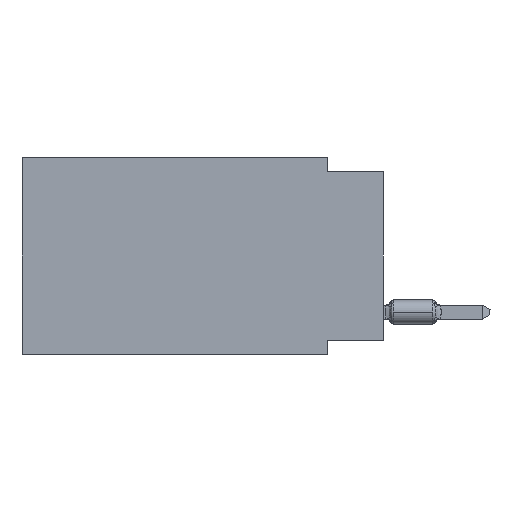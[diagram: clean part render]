
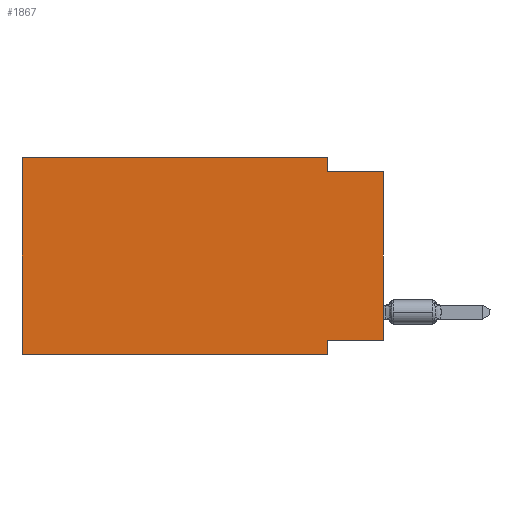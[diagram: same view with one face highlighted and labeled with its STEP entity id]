
A CAD part, left-side view. The second image highlights one B-rep face of the part: STEP entity #1867.
In plain terms, the highlighted planar face has unit normal (-1, 0, 0).
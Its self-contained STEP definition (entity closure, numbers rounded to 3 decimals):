
#154 = LINE ( 'NONE', #67499, #51391 ) ;
#655 = CARTESIAN_POINT ( 'NONE',  ( 0., 2.54, -0.635 ) ) ;
#1867 = ADVANCED_FACE ( 'NONE', ( #7643 ), #2832, .F. ) ;
#2832 = PLANE ( 'NONE',  #65739 ) ;
#3034 = EDGE_CURVE ( 'NONE', #3789, #51881, #59433, .T. ) ;
#3789 = VERTEX_POINT ( 'NONE', #67190 ) ;
#3911 = DIRECTION ( 'NONE',  ( 0., -1., 0. ) ) ;
#4207 = DIRECTION ( 'NONE',  ( 0., -1., 0. ) ) ;
#5122 = CARTESIAN_POINT ( 'NONE',  ( 0., 16.383, 0. ) ) ;
#7643 = FACE_OUTER_BOUND ( 'NONE', #57859, .T. ) ;
#7792 = EDGE_CURVE ( 'NONE', #61002, #53414, #52533, .T. ) ;
#8003 = EDGE_CURVE ( 'NONE', #22742, #40839, #56196, .T. ) ;
#10367 = VECTOR ( 'NONE', #4207, 1000. ) ;
#12188 = EDGE_CURVE ( 'NONE', #40839, #38805, #57077, .T. ) ;
#13279 = VECTOR ( 'NONE', #58087, 1000. ) ;
#13514 = CARTESIAN_POINT ( 'NONE',  ( 0., 16.383, 0. ) ) ;
#16881 = ORIENTED_EDGE ( 'NONE', *, *, #3034, .T. ) ;
#18961 = CARTESIAN_POINT ( 'NONE',  ( 0., 2.54, 0. ) ) ;
#22253 = DIRECTION ( 'NONE',  ( 0., 0., 1. ) ) ;
#22742 = VERTEX_POINT ( 'NONE', #44906 ) ;
#22993 = CARTESIAN_POINT ( 'NONE',  ( 0., 2.54, -8.89 ) ) ;
#23925 = CARTESIAN_POINT ( 'NONE',  ( 0., 0., -0.635 ) ) ;
#24015 = EDGE_CURVE ( 'NONE', #38805, #30561, #26499, .T. ) ;
#26151 = CARTESIAN_POINT ( 'NONE',  ( 0., 2.54, 0. ) ) ;
#26499 = LINE ( 'NONE', #26151, #55905 ) ;
#29197 = ORIENTED_EDGE ( 'NONE', *, *, #32915, .F. ) ;
#30561 = VERTEX_POINT ( 'NONE', #655 ) ;
#32915 = EDGE_CURVE ( 'NONE', #30561, #51881, #44941, .T. ) ;
#32962 = CARTESIAN_POINT ( 'NONE',  ( 0., 16.383, 0. ) ) ;
#33494 = CARTESIAN_POINT ( 'NONE',  ( 0., 0., 0. ) ) ;
#38802 = EDGE_CURVE ( 'NONE', #22742, #53414, #51077, .T. ) ;
#38805 = VERTEX_POINT ( 'NONE', #18961 ) ;
#40839 = VERTEX_POINT ( 'NONE', #63967 ) ;
#41235 = CARTESIAN_POINT ( 'NONE',  ( 0., 2.54, -8.89 ) ) ;
#41567 = CARTESIAN_POINT ( 'NONE',  ( 0., 2.54, -8.255 ) ) ;
#41884 = DIRECTION ( 'NONE',  ( 0., 1., 0. ) ) ;
#42263 = DIRECTION ( 'NONE',  ( 0., 0., -1. ) ) ;
#42413 = VECTOR ( 'NONE', #42263, 1000. ) ;
#43211 = DIRECTION ( 'NONE',  ( 1., 0., 0. ) ) ;
#44906 = CARTESIAN_POINT ( 'NONE',  ( 0., 16.383, -8.89 ) ) ;
#44941 = LINE ( 'NONE', #65782, #63286 ) ;
#46166 = ORIENTED_EDGE ( 'NONE', *, *, #8003, .F. ) ;
#46288 = DIRECTION ( 'NONE',  ( 0., 0., -1. ) ) ;
#51077 = LINE ( 'NONE', #60277, #10367 ) ;
#51214 = VECTOR ( 'NONE', #56529, 1000. ) ;
#51391 = VECTOR ( 'NONE', #41884, 1000. ) ;
#51881 = VERTEX_POINT ( 'NONE', #23925 ) ;
#52533 = LINE ( 'NONE', #41235, #42413 ) ;
#53342 = ORIENTED_EDGE ( 'NONE', *, *, #7792, .F. ) ;
#53414 = VERTEX_POINT ( 'NONE', #22993 ) ;
#53476 = ORIENTED_EDGE ( 'NONE', *, *, #12188, .F. ) ;
#55905 = VECTOR ( 'NONE', #46288, 1000. ) ;
#56196 = LINE ( 'NONE', #13514, #51214 ) ;
#56529 = DIRECTION ( 'NONE',  ( 0., 0., 1. ) ) ;
#57077 = LINE ( 'NONE', #5122, #13279 ) ;
#57480 = EDGE_CURVE ( 'NONE', #3789, #61002, #154, .T. ) ;
#57859 = EDGE_LOOP ( 'NONE', ( #16881, #29197, #62377, #53476, #46166, #60210, #53342, #62595 ) ) ;
#58087 = DIRECTION ( 'NONE',  ( 0., -1., 0. ) ) ;
#59433 = LINE ( 'NONE', #33494, #61640 ) ;
#60210 = ORIENTED_EDGE ( 'NONE', *, *, #38802, .T. ) ;
#60277 = CARTESIAN_POINT ( 'NONE',  ( 0., 16.383, -8.89 ) ) ;
#61002 = VERTEX_POINT ( 'NONE', #41567 ) ;
#61640 = VECTOR ( 'NONE', #22253, 1000. ) ;
#62377 = ORIENTED_EDGE ( 'NONE', *, *, #24015, .F. ) ;
#62595 = ORIENTED_EDGE ( 'NONE', *, *, #57480, .F. ) ;
#63286 = VECTOR ( 'NONE', #3911, 1000. ) ;
#63967 = CARTESIAN_POINT ( 'NONE',  ( 0., 16.383, 0. ) ) ;
#64382 = DIRECTION ( 'NONE',  ( 0., 0., -1. ) ) ;
#65739 = AXIS2_PLACEMENT_3D ( 'NONE', #32962, #43211, #64382 ) ;
#65782 = CARTESIAN_POINT ( 'NONE',  ( 0., 0., -0.635 ) ) ;
#67190 = CARTESIAN_POINT ( 'NONE',  ( 0., 0., -8.255 ) ) ;
#67499 = CARTESIAN_POINT ( 'NONE',  ( 0., 0., -8.255 ) ) ;
